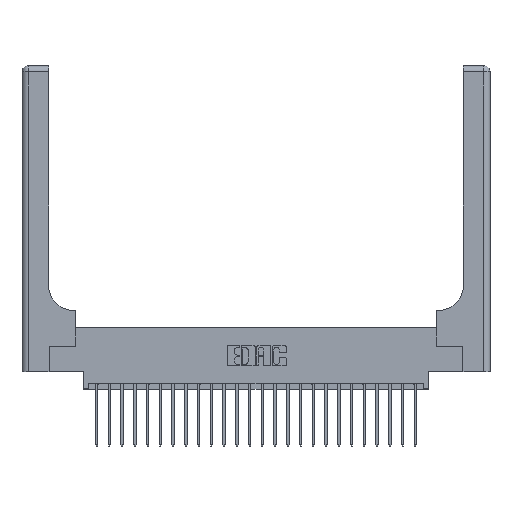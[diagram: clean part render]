
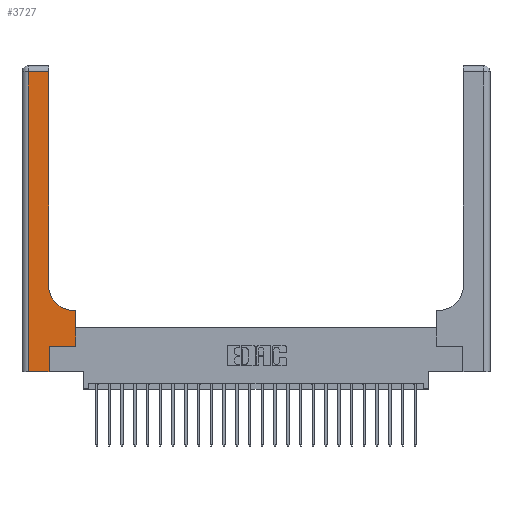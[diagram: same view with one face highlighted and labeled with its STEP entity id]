
A CAD part, top view. The second image highlights one B-rep face of the part: STEP entity #3727.
In plain terms, the highlighted planar face has unit normal (0, 0, 1).
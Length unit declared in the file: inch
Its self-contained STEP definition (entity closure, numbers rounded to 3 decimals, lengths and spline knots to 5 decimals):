
#22 = VERTEX_POINT ( 'NONE', #4549 ) ;
#54 = ORIENTED_EDGE ( 'NONE', *, *, #24305, .T. ) ;
#56 = EDGE_CURVE ( 'NONE', #8016, #22, #17993, .T. ) ;
#257 = FACE_OUTER_BOUND ( 'NONE', #17706, .T. ) ;
#302 = VECTOR ( 'NONE', #8689, 39.37008 ) ;
#1206 = DIRECTION ( 'NONE',  ( 0., 1., 0. ) ) ;
#1367 = CARTESIAN_POINT ( 'NONE',  ( 0.51, 0.85, 0.37 ) ) ;
#2576 = VERTEX_POINT ( 'NONE', #13245 ) ;
#2813 = CARTESIAN_POINT ( 'NONE',  ( 0.265, 0., 0.37 ) ) ;
#3261 = ORIENTED_EDGE ( 'NONE', *, *, #4229, .T. ) ;
#3368 = DIRECTION ( 'NONE',  ( 1., 0., 0. ) ) ;
#3727 = ADVANCED_FACE ( 'NONE', ( #257 ), #16542, .F. ) ;
#4046 = EDGE_CURVE ( 'NONE', #22, #10241, #21571, .T. ) ;
#4171 = DIRECTION ( 'NONE',  ( 1., 0., 0. ) ) ;
#4229 = EDGE_CURVE ( 'NONE', #14401, #23062, #15488, .T. ) ;
#4333 = CARTESIAN_POINT ( 'NONE',  ( 0.265, 0.25, 0.37 ) ) ;
#4549 = CARTESIAN_POINT ( 'NONE',  ( 0.528, 0.25, 0.37 ) ) ;
#4794 = DIRECTION ( 'NONE',  ( 0., 1., 0. ) ) ;
#4921 = ORIENTED_EDGE ( 'NONE', *, *, #4046, .T. ) ;
#5281 = LINE ( 'NONE', #12651, #14699 ) ;
#5672 = VERTEX_POINT ( 'NONE', #24223 ) ;
#5683 = CARTESIAN_POINT ( 'NONE',  ( 0.265, 0.25, 0.37 ) ) ;
#6158 = LINE ( 'NONE', #6787, #302 ) ;
#6787 = CARTESIAN_POINT ( 'NONE',  ( 0.06, 3., 0.37 ) ) ;
#7120 = EDGE_CURVE ( 'NONE', #21417, #8016, #9623, .T. ) ;
#7317 = ORIENTED_EDGE ( 'NONE', *, *, #16224, .T. ) ;
#7591 = AXIS2_PLACEMENT_3D ( 'NONE', #14671, #18329, #18403 ) ;
#7786 = CIRCLE ( 'NONE', #17264, 0.25 ) ;
#8016 = VERTEX_POINT ( 'NONE', #5683 ) ;
#8046 = VECTOR ( 'NONE', #4171, 39.37008 ) ;
#8258 = LINE ( 'NONE', #22075, #12671 ) ;
#8594 = CARTESIAN_POINT ( 'NONE',  ( 0.26, 0.85, 0.37 ) ) ;
#8689 = DIRECTION ( 'NONE',  ( 0., -1., 0. ) ) ;
#8803 = VECTOR ( 'NONE', #9822, 39.37008 ) ;
#8870 = ORIENTED_EDGE ( 'NONE', *, *, #7120, .T. ) ;
#9623 = LINE ( 'NONE', #2813, #18969 ) ;
#9822 = DIRECTION ( 'NONE',  ( -1., 0., 0. ) ) ;
#10241 = VERTEX_POINT ( 'NONE', #21122 ) ;
#10256 = DIRECTION ( 'NONE',  ( 0., 1., 0. ) ) ;
#10503 = ORIENTED_EDGE ( 'NONE', *, *, #11121, .T. ) ;
#11121 = EDGE_CURVE ( 'NONE', #10241, #12322, #5281, .T. ) ;
#11701 = VECTOR ( 'NONE', #10256, 39.37008 ) ;
#12170 = EDGE_CURVE ( 'NONE', #23062, #5672, #23681, .T. ) ;
#12322 = VERTEX_POINT ( 'NONE', #13366 ) ;
#12610 = CARTESIAN_POINT ( 'NONE',  ( 0.26, 2.94, 0.37 ) ) ;
#12651 = CARTESIAN_POINT ( 'NONE',  ( 0.26, 0.6, 0.37 ) ) ;
#12671 = VECTOR ( 'NONE', #20200, 39.37008 ) ;
#13245 = CARTESIAN_POINT ( 'NONE',  ( 0.06, 0., 0.37 ) ) ;
#13366 = CARTESIAN_POINT ( 'NONE',  ( 0.51, 0.6, 0.37 ) ) ;
#13720 = VECTOR ( 'NONE', #1206, 39.37008 ) ;
#14214 = ORIENTED_EDGE ( 'NONE', *, *, #56, .T. ) ;
#14401 = VERTEX_POINT ( 'NONE', #8594 ) ;
#14538 = DIRECTION ( 'NONE',  ( -1., 0., 0. ) ) ;
#14671 = CARTESIAN_POINT ( 'NONE',  ( 0., 3., 0.37 ) ) ;
#14699 = VECTOR ( 'NONE', #14538, 39.37008 ) ;
#14710 = DIRECTION ( 'NONE',  ( 0., 0., -1. ) ) ;
#15488 = LINE ( 'NONE', #21941, #13720 ) ;
#16224 = EDGE_CURVE ( 'NONE', #5672, #2576, #6158, .T. ) ;
#16542 = PLANE ( 'NONE',  #7591 ) ;
#17264 = AXIS2_PLACEMENT_3D ( 'NONE', #1367, #14710, #3368 ) ;
#17706 = EDGE_LOOP ( 'NONE', ( #3261, #21302, #7317, #22958, #8870, #14214, #4921, #10503, #54 ) ) ;
#17993 = LINE ( 'NONE', #4333, #8046 ) ;
#18329 = DIRECTION ( 'NONE',  ( 0., 0., -1. ) ) ;
#18403 = DIRECTION ( 'NONE',  ( -1., 0., 0. ) ) ;
#18969 = VECTOR ( 'NONE', #4794, 39.37008 ) ;
#19440 = CARTESIAN_POINT ( 'NONE',  ( 0.265, 0., 0.37 ) ) ;
#19543 = CARTESIAN_POINT ( 'NONE',  ( 0.528, 0.25, 0.37 ) ) ;
#20200 = DIRECTION ( 'NONE',  ( 1., 0., 0. ) ) ;
#20681 = EDGE_CURVE ( 'NONE', #2576, #21417, #8258, .T. ) ;
#21122 = CARTESIAN_POINT ( 'NONE',  ( 0.528, 0.6, 0.37 ) ) ;
#21302 = ORIENTED_EDGE ( 'NONE', *, *, #12170, .T. ) ;
#21417 = VERTEX_POINT ( 'NONE', #19440 ) ;
#21571 = LINE ( 'NONE', #19543, #11701 ) ;
#21941 = CARTESIAN_POINT ( 'NONE',  ( 0.26, 3., 0.37 ) ) ;
#22075 = CARTESIAN_POINT ( 'NONE',  ( 0., 0., 0.37 ) ) ;
#22854 = CARTESIAN_POINT ( 'NONE',  ( 0., 2.94, 0.37 ) ) ;
#22958 = ORIENTED_EDGE ( 'NONE', *, *, #20681, .T. ) ;
#23062 = VERTEX_POINT ( 'NONE', #12610 ) ;
#23681 = LINE ( 'NONE', #22854, #8803 ) ;
#24223 = CARTESIAN_POINT ( 'NONE',  ( 0.06, 2.94, 0.37 ) ) ;
#24305 = EDGE_CURVE ( 'NONE', #12322, #14401, #7786, .T. ) ;
